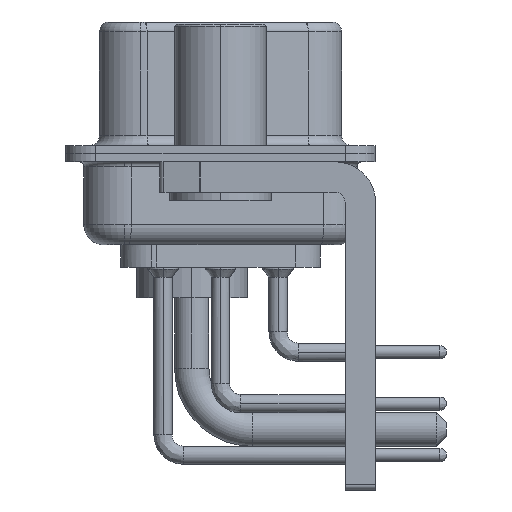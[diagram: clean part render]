
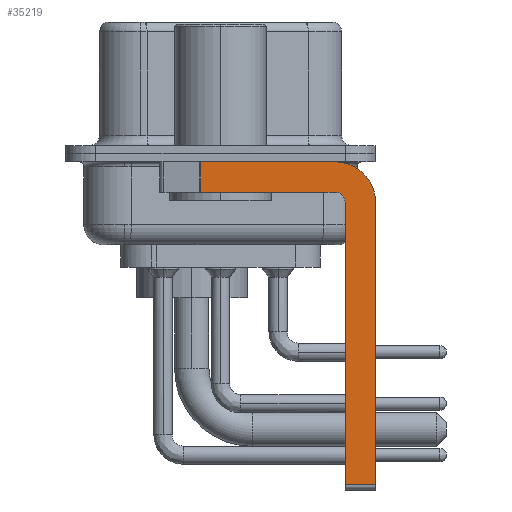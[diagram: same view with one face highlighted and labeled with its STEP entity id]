
A CAD part, left-side view. The second image highlights one B-rep face of the part: STEP entity #35219.
In plain terms, the highlighted planar face has unit normal (-1, 0, 0).
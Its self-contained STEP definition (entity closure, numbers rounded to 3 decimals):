
#624 = VECTOR ( 'NONE', #4585, 1000. ) ;
#1416 = DIRECTION ( 'NONE',  ( -1., 0., 0. ) ) ;
#2249 = DIRECTION ( 'NONE',  ( 0., 0., -1. ) ) ;
#2455 = VERTEX_POINT ( 'NONE', #24546 ) ;
#2894 = LINE ( 'NONE', #11697, #14996 ) ;
#3266 = VERTEX_POINT ( 'NONE', #9885 ) ;
#3297 = VERTEX_POINT ( 'NONE', #20046 ) ;
#4236 = EDGE_LOOP ( 'NONE', ( #27680, #15696, #6917, #4575, #11795, #38120, #6704, #22235 ) ) ;
#4575 = ORIENTED_EDGE ( 'NONE', *, *, #5094, .F. ) ;
#4585 = DIRECTION ( 'NONE',  ( 0., 1., 0. ) ) ;
#5094 = EDGE_CURVE ( 'NONE', #2455, #33035, #12968, .T. ) ;
#5188 = LINE ( 'NONE', #35562, #35258 ) ;
#5750 = VERTEX_POINT ( 'NONE', #34138 ) ;
#6005 = VECTOR ( 'NONE', #12925, 1000. ) ;
#6085 = EDGE_CURVE ( 'NONE', #20310, #3297, #9292, .T. ) ;
#6704 = ORIENTED_EDGE ( 'NONE', *, *, #22628, .F. ) ;
#6826 = VECTOR ( 'NONE', #9696, 1000. ) ;
#6917 = ORIENTED_EDGE ( 'NONE', *, *, #22750, .F. ) ;
#9292 = CIRCLE ( 'NONE', #18726, 2. ) ;
#9576 = CARTESIAN_POINT ( 'NONE',  ( -2.9, -5.65, -1.9 ) ) ;
#9696 = DIRECTION ( 'NONE',  ( 0., 0., -1. ) ) ;
#9885 = CARTESIAN_POINT ( 'NONE',  ( -2.9, -6.15, -16.35 ) ) ;
#11004 = VECTOR ( 'NONE', #2249, 1000. ) ;
#11119 = AXIS2_PLACEMENT_3D ( 'NONE', #16518, #1416, #22423 ) ;
#11697 = CARTESIAN_POINT ( 'NONE',  ( -2.9, 3., -0.4 ) ) ;
#11795 = ORIENTED_EDGE ( 'NONE', *, *, #30710, .F. ) ;
#12925 = DIRECTION ( 'NONE',  ( 0., -1., 0. ) ) ;
#12968 = CIRCLE ( 'NONE', #11119, 0.5 ) ;
#14996 = VECTOR ( 'NONE', #20952, 1000. ) ;
#15696 = ORIENTED_EDGE ( 'NONE', *, *, #17742, .T. ) ;
#16013 = VERTEX_POINT ( 'NONE', #36617 ) ;
#16518 = CARTESIAN_POINT ( 'NONE',  ( -2.9, -5.65, -2.4 ) ) ;
#17742 = EDGE_CURVE ( 'NONE', #16013, #22490, #19925, .T. ) ;
#17962 = CARTESIAN_POINT ( 'NONE',  ( -2.9, -7.65, -2.4 ) ) ;
#18726 = AXIS2_PLACEMENT_3D ( 'NONE', #32881, #30335, #21321 ) ;
#19521 = CARTESIAN_POINT ( 'NONE',  ( -2.9, -5.65, -1.9 ) ) ;
#19712 = LINE ( 'NONE', #19521, #624 ) ;
#19925 = LINE ( 'NONE', #28943, #11004 ) ;
#20046 = CARTESIAN_POINT ( 'NONE',  ( -2.9, -7.65, -2.4 ) ) ;
#20310 = VERTEX_POINT ( 'NONE', #23938 ) ;
#20697 = DIRECTION ( 'NONE',  ( 0., 0., 1. ) ) ;
#20952 = DIRECTION ( 'NONE',  ( 0., -1., 0. ) ) ;
#21321 = DIRECTION ( 'NONE',  ( 0., 0., -1. ) ) ;
#22235 = ORIENTED_EDGE ( 'NONE', *, *, #6085, .F. ) ;
#22423 = DIRECTION ( 'NONE',  ( 0., 0., 1. ) ) ;
#22490 = VERTEX_POINT ( 'NONE', #26214 ) ;
#22628 = EDGE_CURVE ( 'NONE', #3297, #5750, #30312, .T. ) ;
#22750 = EDGE_CURVE ( 'NONE', #33035, #22490, #19712, .T. ) ;
#23938 = CARTESIAN_POINT ( 'NONE',  ( -2.9, -5.65, -0.4 ) ) ;
#24546 = CARTESIAN_POINT ( 'NONE',  ( -2.9, -6.15, -2.4 ) ) ;
#26214 = CARTESIAN_POINT ( 'NONE',  ( -2.9, 0.978, -1.9 ) ) ;
#27680 = ORIENTED_EDGE ( 'NONE', *, *, #38517, .F. ) ;
#28396 = PLANE ( 'NONE',  #31719 ) ;
#28943 = CARTESIAN_POINT ( 'NONE',  ( -2.9, 0.978, -1.9 ) ) ;
#29159 = CARTESIAN_POINT ( 'NONE',  ( -2.9, -5.65, -2.4 ) ) ;
#30312 = LINE ( 'NONE', #17962, #6826 ) ;
#30335 = DIRECTION ( 'NONE',  ( 1., 0., 0. ) ) ;
#30710 = EDGE_CURVE ( 'NONE', #3266, #2455, #5188, .T. ) ;
#31709 = DIRECTION ( 'NONE',  ( 0., 0., -1. ) ) ;
#31719 = AXIS2_PLACEMENT_3D ( 'NONE', #29159, #37960, #31709 ) ;
#32081 = FACE_OUTER_BOUND ( 'NONE', #4236, .T. ) ;
#32881 = CARTESIAN_POINT ( 'NONE',  ( -2.9, -5.65, -2.4 ) ) ;
#33035 = VERTEX_POINT ( 'NONE', #9576 ) ;
#33529 = CARTESIAN_POINT ( 'NONE',  ( -2.9, -5.65, -16.35 ) ) ;
#34138 = CARTESIAN_POINT ( 'NONE',  ( -2.9, -7.65, -16.35 ) ) ;
#34861 = EDGE_CURVE ( 'NONE', #3266, #5750, #36461, .T. ) ;
#35219 = ADVANCED_FACE ( 'NONE', ( #32081 ), #28396, .F. ) ;
#35258 = VECTOR ( 'NONE', #20697, 1000. ) ;
#35562 = CARTESIAN_POINT ( 'NONE',  ( -2.9, -6.15, -16.6 ) ) ;
#36461 = LINE ( 'NONE', #33529, #6005 ) ;
#36617 = CARTESIAN_POINT ( 'NONE',  ( -2.9, 0.978, -0.4 ) ) ;
#37960 = DIRECTION ( 'NONE',  ( 1., 0., 0. ) ) ;
#38120 = ORIENTED_EDGE ( 'NONE', *, *, #34861, .T. ) ;
#38517 = EDGE_CURVE ( 'NONE', #16013, #20310, #2894, .T. ) ;
